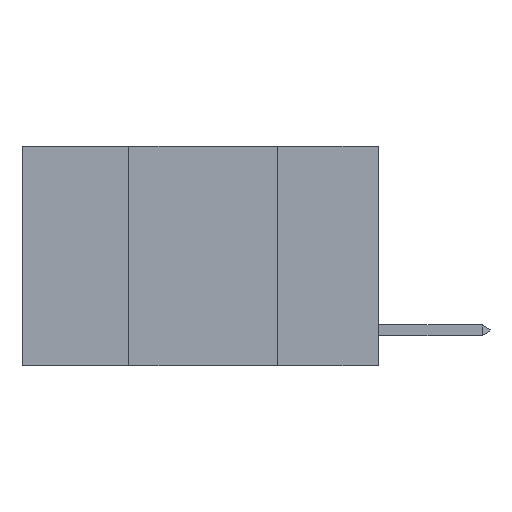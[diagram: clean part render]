
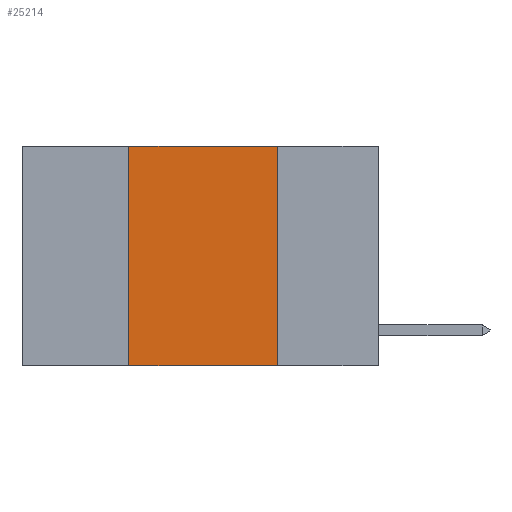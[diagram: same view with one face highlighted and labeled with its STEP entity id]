
A CAD part, left-side view. The second image highlights one B-rep face of the part: STEP entity #25214.
In plain terms, the highlighted planar face has unit normal (-1, 0, 0).
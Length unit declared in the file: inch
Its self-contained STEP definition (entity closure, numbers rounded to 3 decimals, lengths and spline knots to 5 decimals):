
#780 = CARTESIAN_POINT ( 'NONE',  ( 0., 0.42, 0. ) ) ;
#1452 = AXIS2_PLACEMENT_3D ( 'NONE', #18222, #20333, #11443 ) ;
#1882 = EDGE_CURVE ( 'NONE', #8819, #8639, #29455, .T. ) ;
#2350 = CARTESIAN_POINT ( 'NONE',  ( 0., 0.6, -0.37 ) ) ;
#2866 = CARTESIAN_POINT ( 'NONE',  ( 0., 0.42, 0. ) ) ;
#3123 = EDGE_CURVE ( 'NONE', #8639, #19324, #15501, .T. ) ;
#6167 = VECTOR ( 'NONE', #8281, 39.37008 ) ;
#8202 = VECTOR ( 'NONE', #20705, 39.37008 ) ;
#8281 = DIRECTION ( 'NONE',  ( 0., 0., -1. ) ) ;
#8639 = VERTEX_POINT ( 'NONE', #20606 ) ;
#8819 = VERTEX_POINT ( 'NONE', #2866 ) ;
#8824 = DIRECTION ( 'NONE',  ( 0., -1., 0. ) ) ;
#9706 = ORIENTED_EDGE ( 'NONE', *, *, #11767, .T. ) ;
#9856 = VERTEX_POINT ( 'NONE', #15653 ) ;
#10000 = VECTOR ( 'NONE', #8824, 39.37008 ) ;
#11443 = DIRECTION ( 'NONE',  ( 0., 0., -1. ) ) ;
#11767 = EDGE_CURVE ( 'NONE', #9856, #19324, #16037, .T. ) ;
#14309 = LINE ( 'NONE', #780, #25766 ) ;
#15501 = LINE ( 'NONE', #22710, #6167 ) ;
#15653 = CARTESIAN_POINT ( 'NONE',  ( 0., 0.42, -0.37 ) ) ;
#16037 = LINE ( 'NONE', #2350, #8202 ) ;
#18222 = CARTESIAN_POINT ( 'NONE',  ( 0., 0.6, 0. ) ) ;
#19324 = VERTEX_POINT ( 'NONE', #22193 ) ;
#20121 = CARTESIAN_POINT ( 'NONE',  ( 0., 0.6, 0. ) ) ;
#20333 = DIRECTION ( 'NONE',  ( 1., 0., 0. ) ) ;
#20606 = CARTESIAN_POINT ( 'NONE',  ( 0., 0.17, 0. ) ) ;
#20705 = DIRECTION ( 'NONE',  ( 0., -1., 0. ) ) ;
#21428 = EDGE_CURVE ( 'NONE', #9856, #8819, #14309, .T. ) ;
#21569 = ORIENTED_EDGE ( 'NONE', *, *, #21428, .F. ) ;
#22193 = CARTESIAN_POINT ( 'NONE',  ( 0., 0.17, -0.37 ) ) ;
#22710 = CARTESIAN_POINT ( 'NONE',  ( 0., 0.17, 0. ) ) ;
#23172 = ORIENTED_EDGE ( 'NONE', *, *, #1882, .F. ) ;
#23190 = DIRECTION ( 'NONE',  ( 0., 0., 1. ) ) ;
#24251 = EDGE_LOOP ( 'NONE', ( #29574, #23172, #21569, #9706 ) ) ;
#25214 = ADVANCED_FACE ( 'NONE', ( #29510 ), #29365, .F. ) ;
#25766 = VECTOR ( 'NONE', #23190, 39.37008 ) ;
#29365 = PLANE ( 'NONE',  #1452 ) ;
#29455 = LINE ( 'NONE', #20121, #10000 ) ;
#29510 = FACE_OUTER_BOUND ( 'NONE', #24251, .T. ) ;
#29574 = ORIENTED_EDGE ( 'NONE', *, *, #3123, .F. ) ;
